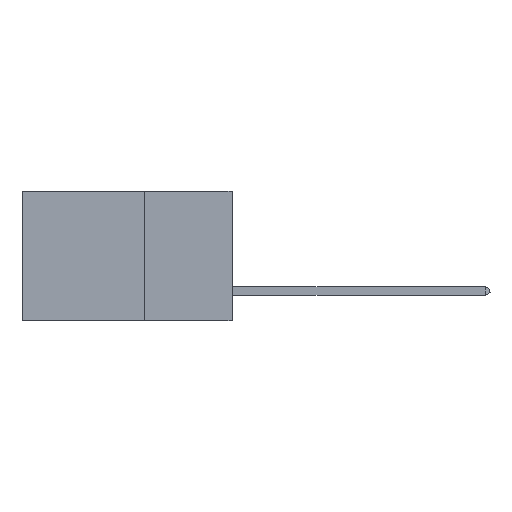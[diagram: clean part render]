
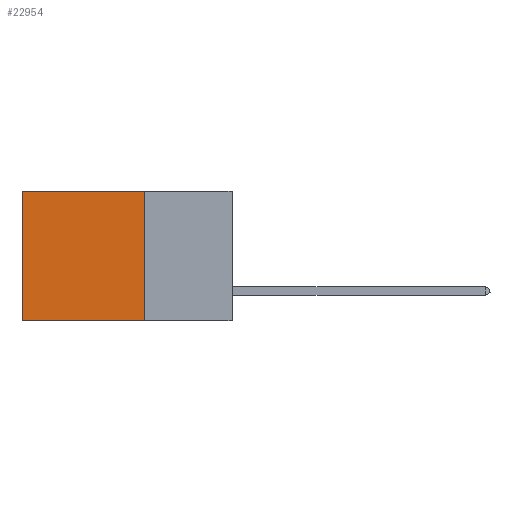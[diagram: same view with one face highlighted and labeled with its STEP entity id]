
A CAD part, left-side view. The second image highlights one B-rep face of the part: STEP entity #22954.
In plain terms, the highlighted planar face has unit normal (-1, 0, 0).
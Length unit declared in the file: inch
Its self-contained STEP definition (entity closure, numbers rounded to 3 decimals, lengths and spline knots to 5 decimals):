
#303 = EDGE_LOOP ( 'NONE', ( #4266, #24906, #14605, #20119 ) ) ;
#1062 = AXIS2_PLACEMENT_3D ( 'NONE', #10749, #29107, #22297 ) ;
#1690 = PLANE ( 'NONE',  #1062 ) ;
#1741 = LINE ( 'NONE', #3259, #29059 ) ;
#2716 = DIRECTION ( 'NONE',  ( 0., 0., -1. ) ) ;
#3259 = CARTESIAN_POINT ( 'NONE',  ( 0.2875, 0.6, 0. ) ) ;
#3350 = EDGE_CURVE ( 'NONE', #15251, #17449, #1741, .T. ) ;
#4266 = ORIENTED_EDGE ( 'NONE', *, *, #3350, .T. ) ;
#4604 = CARTESIAN_POINT ( 'NONE',  ( 0.2875, 0.25, -0.37 ) ) ;
#7439 = CARTESIAN_POINT ( 'NONE',  ( 0.2875, 0.25, 0. ) ) ;
#7629 = CARTESIAN_POINT ( 'NONE',  ( 0.2875, 0.6, 0. ) ) ;
#8362 = LINE ( 'NONE', #16756, #15197 ) ;
#10749 = CARTESIAN_POINT ( 'NONE',  ( 0.2875, 0.25, 0. ) ) ;
#10943 = FACE_OUTER_BOUND ( 'NONE', #303, .T. ) ;
#11091 = LINE ( 'NONE', #7439, #18628 ) ;
#14605 = ORIENTED_EDGE ( 'NONE', *, *, #27211, .F. ) ;
#14608 = DIRECTION ( 'NONE',  ( 0., 1., 0. ) ) ;
#15197 = VECTOR ( 'NONE', #16940, 39.37008 ) ;
#15251 = VERTEX_POINT ( 'NONE', #7629 ) ;
#16756 = CARTESIAN_POINT ( 'NONE',  ( 0.2875, 0.25, 0. ) ) ;
#16940 = DIRECTION ( 'NONE',  ( 0., 1., 0. ) ) ;
#17449 = VERTEX_POINT ( 'NONE', #19663 ) ;
#18628 = VECTOR ( 'NONE', #2716, 39.37008 ) ;
#19136 = CARTESIAN_POINT ( 'NONE',  ( 0.2875, 0.25, -0.37 ) ) ;
#19663 = CARTESIAN_POINT ( 'NONE',  ( 0.2875, 0.6, -0.37 ) ) ;
#20119 = ORIENTED_EDGE ( 'NONE', *, *, #23468, .T. ) ;
#22297 = DIRECTION ( 'NONE',  ( 0., 0., -1. ) ) ;
#22954 = ADVANCED_FACE ( 'NONE', ( #10943 ), #1690, .F. ) ;
#23321 = VECTOR ( 'NONE', #14608, 39.37008 ) ;
#23468 = EDGE_CURVE ( 'NONE', #25525, #15251, #8362, .T. ) ;
#23699 = CARTESIAN_POINT ( 'NONE',  ( 0.2875, 0.25, 0. ) ) ;
#24056 = DIRECTION ( 'NONE',  ( 0., 0., -1. ) ) ;
#24906 = ORIENTED_EDGE ( 'NONE', *, *, #25069, .F. ) ;
#25069 = EDGE_CURVE ( 'NONE', #27674, #17449, #26584, .T. ) ;
#25525 = VERTEX_POINT ( 'NONE', #23699 ) ;
#26584 = LINE ( 'NONE', #19136, #23321 ) ;
#27211 = EDGE_CURVE ( 'NONE', #25525, #27674, #11091, .T. ) ;
#27674 = VERTEX_POINT ( 'NONE', #4604 ) ;
#29059 = VECTOR ( 'NONE', #24056, 39.37008 ) ;
#29107 = DIRECTION ( 'NONE',  ( 1., 0., 0. ) ) ;
